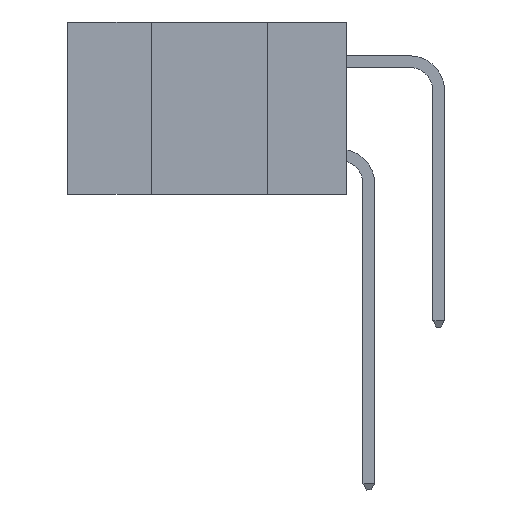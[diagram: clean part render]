
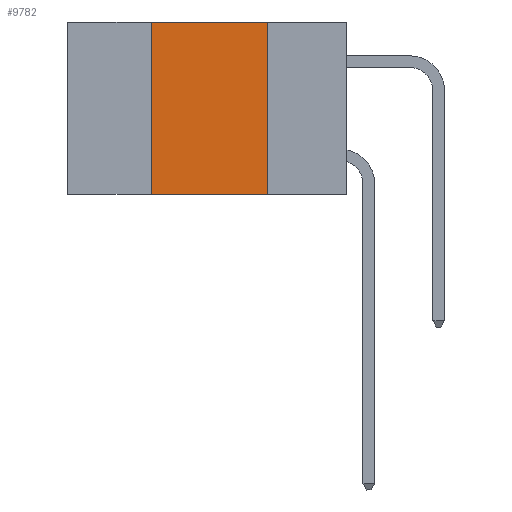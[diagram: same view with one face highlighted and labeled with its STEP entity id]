
A CAD part, left-side view. The second image highlights one B-rep face of the part: STEP entity #9782.
In plain terms, the highlighted planar face has unit normal (-1, 0, 0).
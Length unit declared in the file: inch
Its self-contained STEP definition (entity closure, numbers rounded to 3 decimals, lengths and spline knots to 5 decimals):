
#131 = LINE ( 'NONE', #5772, #8412 ) ;
#221 = CARTESIAN_POINT ( 'NONE',  ( 0., 0.42, 0. ) ) ;
#317 = EDGE_LOOP ( 'NONE', ( #3918, #10891, #634, #537 ) ) ;
#471 = CARTESIAN_POINT ( 'NONE',  ( 0., 0.17, 0. ) ) ;
#503 = VECTOR ( 'NONE', #1360, 39.37008 ) ;
#537 = ORIENTED_EDGE ( 'NONE', *, *, #782, .T. ) ;
#619 = VECTOR ( 'NONE', #9120, 39.37008 ) ;
#634 = ORIENTED_EDGE ( 'NONE', *, *, #6239, .F. ) ;
#782 = EDGE_CURVE ( 'NONE', #1991, #2712, #131, .T. ) ;
#1360 = DIRECTION ( 'NONE',  ( 0., -1., 0. ) ) ;
#1991 = VERTEX_POINT ( 'NONE', #4639 ) ;
#2712 = VERTEX_POINT ( 'NONE', #5130 ) ;
#2921 = CARTESIAN_POINT ( 'NONE',  ( 0., 0.42, 0. ) ) ;
#3178 = PLANE ( 'NONE',  #6491 ) ;
#3918 = ORIENTED_EDGE ( 'NONE', *, *, #6315, .F. ) ;
#4183 = CARTESIAN_POINT ( 'NONE',  ( 0., 0.17, 0. ) ) ;
#4349 = EDGE_CURVE ( 'NONE', #7238, #8849, #8309, .T. ) ;
#4634 = CARTESIAN_POINT ( 'NONE',  ( 0., 0.6, 0. ) ) ;
#4639 = CARTESIAN_POINT ( 'NONE',  ( 0., 0.42, -0.37 ) ) ;
#4754 = VECTOR ( 'NONE', #12003, 39.37008 ) ;
#5130 = CARTESIAN_POINT ( 'NONE',  ( 0., 0.17, -0.37 ) ) ;
#5190 = LINE ( 'NONE', #221, #4754 ) ;
#5772 = CARTESIAN_POINT ( 'NONE',  ( 0., 0.6, -0.37 ) ) ;
#6198 = CARTESIAN_POINT ( 'NONE',  ( 0., 0.6, 0. ) ) ;
#6239 = EDGE_CURVE ( 'NONE', #1991, #7238, #5190, .T. ) ;
#6315 = EDGE_CURVE ( 'NONE', #8849, #2712, #10231, .T. ) ;
#6491 = AXIS2_PLACEMENT_3D ( 'NONE', #4634, #10338, #11896 ) ;
#7238 = VERTEX_POINT ( 'NONE', #2921 ) ;
#8309 = LINE ( 'NONE', #6198, #503 ) ;
#8412 = VECTOR ( 'NONE', #12615, 39.37008 ) ;
#8849 = VERTEX_POINT ( 'NONE', #471 ) ;
#9120 = DIRECTION ( 'NONE',  ( 0., 0., -1. ) ) ;
#9782 = ADVANCED_FACE ( 'NONE', ( #12171 ), #3178, .F. ) ;
#10231 = LINE ( 'NONE', #4183, #619 ) ;
#10338 = DIRECTION ( 'NONE',  ( 1., 0., 0. ) ) ;
#10891 = ORIENTED_EDGE ( 'NONE', *, *, #4349, .F. ) ;
#11896 = DIRECTION ( 'NONE',  ( 0., 0., -1. ) ) ;
#12003 = DIRECTION ( 'NONE',  ( 0., 0., 1. ) ) ;
#12171 = FACE_OUTER_BOUND ( 'NONE', #317, .T. ) ;
#12615 = DIRECTION ( 'NONE',  ( 0., -1., 0. ) ) ;
